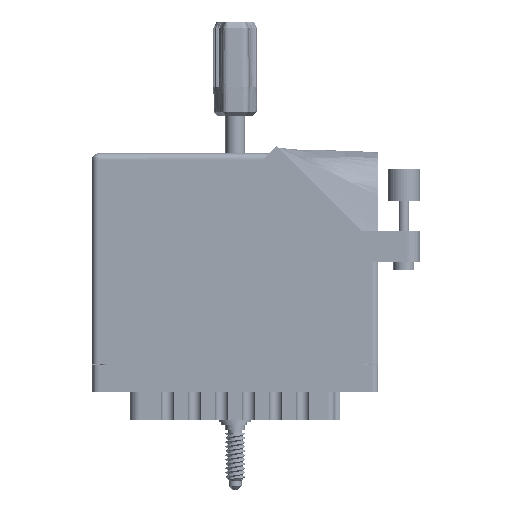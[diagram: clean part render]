
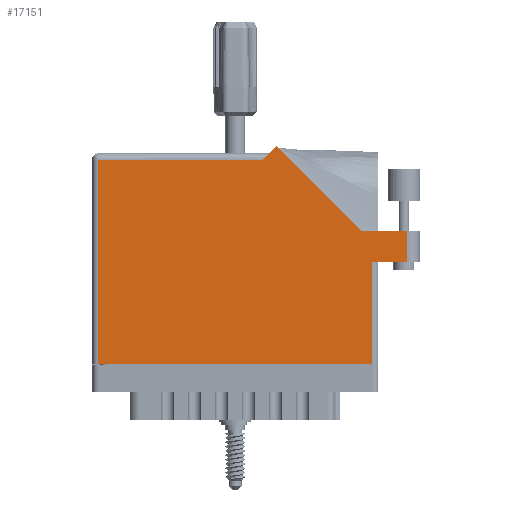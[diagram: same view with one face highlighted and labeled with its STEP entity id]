
A CAD part, front view. The second image highlights one B-rep face of the part: STEP entity #17151.
In plain terms, the highlighted face is planar.
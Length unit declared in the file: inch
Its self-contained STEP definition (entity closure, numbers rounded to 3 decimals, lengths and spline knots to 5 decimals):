
#1499 = CARTESIAN_POINT ( 'NONE',  ( 2.58942, 1.287, 0. ) ) ;
#2960 = DIRECTION ( 'NONE',  ( -0.707, 0.707, 0. ) ) ;
#4805 = DIRECTION ( 'NONE',  ( -1., 0., 0. ) ) ;
#5364 = LINE ( 'NONE', #85364, #19911 ) ;
#6931 = CARTESIAN_POINT ( 'NONE',  ( 3.03, 1.287, 0. ) ) ;
#8282 = VERTEX_POINT ( 'NONE', #37893 ) ;
#10375 = DIRECTION ( 'NONE',  ( 0., 1., 0. ) ) ;
#11313 = ORIENTED_EDGE ( 'NONE', *, *, #64314, .T. ) ;
#11964 = CARTESIAN_POINT ( 'NONE',  ( 3.03, 0.98, 0. ) ) ;
#13509 = AXIS2_PLACEMENT_3D ( 'NONE', #78035, #84745, #101701 ) ;
#14422 = EDGE_CURVE ( 'NONE', #22229, #65387, #88248, .T. ) ;
#16382 = CARTESIAN_POINT ( 'NONE',  ( 0.062, 0., 0. ) ) ;
#17151 = ADVANCED_FACE ( 'NONE', ( #32401 ), #68442, .F. ) ;
#18006 = DIRECTION ( 'NONE',  ( 0., -1., 0. ) ) ;
#18160 = LINE ( 'NONE', #21140, #33986 ) ;
#19911 = VECTOR ( 'NONE', #26622, 39.37008 ) ;
#20465 = VECTOR ( 'NONE', #92258, 39.37008 ) ;
#21140 = CARTESIAN_POINT ( 'NONE',  ( 1.705, 2.03, 0. ) ) ;
#22210 = VECTOR ( 'NONE', #10375, 39.37008 ) ;
#22229 = VERTEX_POINT ( 'NONE', #11964 ) ;
#22714 = LINE ( 'NONE', #1499, #84868 ) ;
#25435 = EDGE_CURVE ( 'NONE', #91402, #76625, #22714, .T. ) ;
#26622 = DIRECTION ( 'NONE',  ( -1., 0., 0. ) ) ;
#30324 = ORIENTED_EDGE ( 'NONE', *, *, #25435, .T. ) ;
#31357 = VECTOR ( 'NONE', #18006, 39.37008 ) ;
#32401 = FACE_OUTER_BOUND ( 'NONE', #49347, .T. ) ;
#33544 = EDGE_CURVE ( 'NONE', #99593, #8282, #99272, .T. ) ;
#33986 = VECTOR ( 'NONE', #63666, 39.37008 ) ;
#34257 = CARTESIAN_POINT ( 'NONE',  ( 0., 0., 0. ) ) ;
#35166 = VECTOR ( 'NONE', #4805, 39.37008 ) ;
#36028 = EDGE_CURVE ( 'NONE', #98135, #99593, #43252, .T. ) ;
#37707 = CARTESIAN_POINT ( 'NONE',  ( 3.155, 1.287, 0. ) ) ;
#37893 = CARTESIAN_POINT ( 'NONE',  ( 2.693, 0., 0. ) ) ;
#40631 = ORIENTED_EDGE ( 'NONE', *, *, #48102, .T. ) ;
#43252 = LINE ( 'NONE', #60208, #31357 ) ;
#46090 = LINE ( 'NONE', #61086, #22210 ) ;
#48102 = EDGE_CURVE ( 'NONE', #87237, #22229, #83913, .T. ) ;
#48984 = ORIENTED_EDGE ( 'NONE', *, *, #51873, .T. ) ;
#49347 = EDGE_LOOP ( 'NONE', ( #40631, #96442, #91615, #30324, #109002, #11313, #94439, #108336, #48984 ) ) ;
#51873 = EDGE_CURVE ( 'NONE', #8282, #87237, #46090, .T. ) ;
#54788 = CARTESIAN_POINT ( 'NONE',  ( 0.062, 1.968, 0. ) ) ;
#55926 = CARTESIAN_POINT ( 'NONE',  ( 1.643, 1.968, 0. ) ) ;
#59581 = VECTOR ( 'NONE', #85593, 39.37008 ) ;
#60090 = CARTESIAN_POINT ( 'NONE',  ( 2.58942, 1.287, 0. ) ) ;
#60208 = CARTESIAN_POINT ( 'NONE',  ( 0.062, 0., 0. ) ) ;
#61086 = CARTESIAN_POINT ( 'NONE',  ( 2.693, 0.98, 0. ) ) ;
#63666 = DIRECTION ( 'NONE',  ( -0.707, -0.707, 0. ) ) ;
#64314 = EDGE_CURVE ( 'NONE', #67827, #98135, #5364, .T. ) ;
#65387 = VERTEX_POINT ( 'NONE', #97126 ) ;
#66824 = DIRECTION ( 'NONE',  ( 0., 1., 0. ) ) ;
#67827 = VERTEX_POINT ( 'NONE', #55926 ) ;
#68442 = PLANE ( 'NONE',  #13509 ) ;
#76625 = VERTEX_POINT ( 'NONE', #80880 ) ;
#78035 = CARTESIAN_POINT ( 'NONE',  ( 0., 2.03, 0. ) ) ;
#80880 = CARTESIAN_POINT ( 'NONE',  ( 1.77571, 2.10071, 0. ) ) ;
#81328 = EDGE_CURVE ( 'NONE', #65387, #91402, #109250, .T. ) ;
#83913 = LINE ( 'NONE', #101873, #20465 ) ;
#84745 = DIRECTION ( 'NONE',  ( 0., 0., -1. ) ) ;
#84868 = VECTOR ( 'NONE', #2960, 39.37008 ) ;
#85364 = CARTESIAN_POINT ( 'NONE',  ( 0., 1.968, 0. ) ) ;
#85593 = DIRECTION ( 'NONE',  ( 1., 0., 0. ) ) ;
#87237 = VERTEX_POINT ( 'NONE', #87429 ) ;
#87429 = CARTESIAN_POINT ( 'NONE',  ( 2.693, 0.98, 0. ) ) ;
#88248 = LINE ( 'NONE', #6931, #102762 ) ;
#91402 = VERTEX_POINT ( 'NONE', #60090 ) ;
#91615 = ORIENTED_EDGE ( 'NONE', *, *, #81328, .T. ) ;
#92258 = DIRECTION ( 'NONE',  ( 1., 0., 0. ) ) ;
#94439 = ORIENTED_EDGE ( 'NONE', *, *, #36028, .T. ) ;
#96442 = ORIENTED_EDGE ( 'NONE', *, *, #14422, .T. ) ;
#97126 = CARTESIAN_POINT ( 'NONE',  ( 3.03, 1.287, 0. ) ) ;
#98135 = VERTEX_POINT ( 'NONE', #54788 ) ;
#99272 = LINE ( 'NONE', #34257, #59581 ) ;
#99593 = VERTEX_POINT ( 'NONE', #16382 ) ;
#99921 = EDGE_CURVE ( 'NONE', #76625, #67827, #18160, .T. ) ;
#101701 = DIRECTION ( 'NONE',  ( -1., 0., 0. ) ) ;
#101873 = CARTESIAN_POINT ( 'NONE',  ( 2.755, 0.98, 0. ) ) ;
#102762 = VECTOR ( 'NONE', #66824, 39.37008 ) ;
#108336 = ORIENTED_EDGE ( 'NONE', *, *, #33544, .T. ) ;
#109002 = ORIENTED_EDGE ( 'NONE', *, *, #99921, .T. ) ;
#109250 = LINE ( 'NONE', #37707, #35166 ) ;
